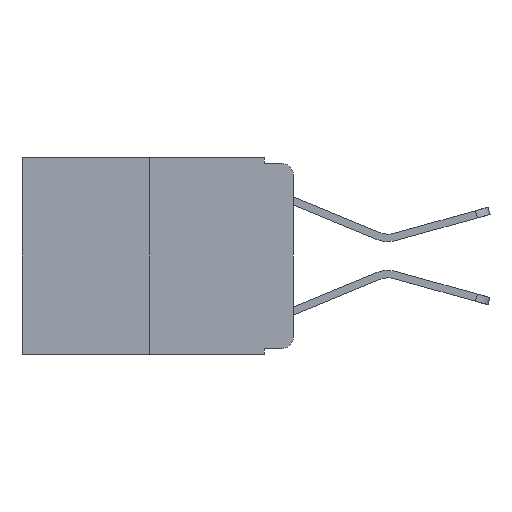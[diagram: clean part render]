
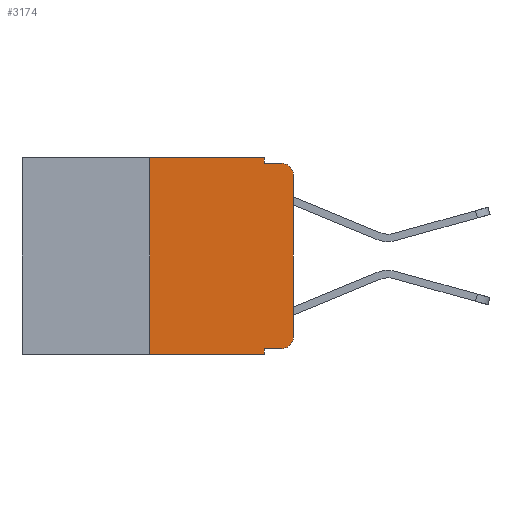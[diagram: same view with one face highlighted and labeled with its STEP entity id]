
A CAD part, left-side view. The second image highlights one B-rep face of the part: STEP entity #3174.
In plain terms, the highlighted planar face has unit normal (-1, 0, 0).
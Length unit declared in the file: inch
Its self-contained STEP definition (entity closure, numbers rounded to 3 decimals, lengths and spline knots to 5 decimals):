
#206 = DIRECTION ( 'NONE',  ( 0., 0., -1. ) ) ;
#505 = ORIENTED_EDGE ( 'NONE', *, *, #9655, .T. ) ;
#578 = VERTEX_POINT ( 'NONE', #1681 ) ;
#584 = CARTESIAN_POINT ( 'NONE',  ( 0., 0.051, -0.343 ) ) ;
#1060 = VERTEX_POINT ( 'NONE', #7971 ) ;
#1079 = LINE ( 'NONE', #1669, #7865 ) ;
#1110 = ORIENTED_EDGE ( 'NONE', *, *, #9670, .T. ) ;
#1277 = VERTEX_POINT ( 'NONE', #584 ) ;
#1289 = VECTOR ( 'NONE', #3260, 39.37008 ) ;
#1319 = DIRECTION ( 'NONE',  ( 0., 0., -1. ) ) ;
#1377 = EDGE_CURVE ( 'NONE', #7410, #1060, #5774, .T. ) ;
#1406 = DIRECTION ( 'NONE',  ( -1., 0., 0. ) ) ;
#1485 = CARTESIAN_POINT ( 'NONE',  ( 0., 0.02, -0.03 ) ) ;
#1519 = VECTOR ( 'NONE', #10667, 39.37008 ) ;
#1527 = CIRCLE ( 'NONE', #7031, 0.02 ) ;
#1564 = LINE ( 'NONE', #7075, #8278 ) ;
#1669 = CARTESIAN_POINT ( 'NONE',  ( 0., 0.051, 0. ) ) ;
#1681 = CARTESIAN_POINT ( 'NONE',  ( 0., 0.051, 0. ) ) ;
#1818 = CARTESIAN_POINT ( 'NONE',  ( 0., 0.02, -0.333 ) ) ;
#2059 = VERTEX_POINT ( 'NONE', #6369 ) ;
#2347 = CARTESIAN_POINT ( 'NONE',  ( 0., 0.02, -0.01 ) ) ;
#2625 = EDGE_CURVE ( 'NONE', #4092, #3668, #1564, .T. ) ;
#2859 = PLANE ( 'NONE',  #4500 ) ;
#3174 = ADVANCED_FACE ( 'NONE', ( #5460 ), #2859, .F. ) ;
#3209 = CARTESIAN_POINT ( 'NONE',  ( 0., 0.051, -0.333 ) ) ;
#3235 = LINE ( 'NONE', #10638, #9751 ) ;
#3260 = DIRECTION ( 'NONE',  ( 0., 0., 1. ) ) ;
#3437 = CIRCLE ( 'NONE', #9424, 0.02 ) ;
#3620 = EDGE_CURVE ( 'NONE', #1060, #3668, #3437, .T. ) ;
#3668 = VERTEX_POINT ( 'NONE', #2347 ) ;
#3849 = EDGE_CURVE ( 'NONE', #578, #4092, #1079, .T. ) ;
#3872 = DIRECTION ( 'NONE',  ( 0., -1., 0. ) ) ;
#4092 = VERTEX_POINT ( 'NONE', #9945 ) ;
#4180 = LINE ( 'NONE', #3209, #8469 ) ;
#4500 = AXIS2_PLACEMENT_3D ( 'NONE', #9171, #6813, #6884 ) ;
#4659 = DIRECTION ( 'NONE',  ( -1., 0., 0. ) ) ;
#4923 = DIRECTION ( 'NONE',  ( 0., -1., 0. ) ) ;
#5192 = ORIENTED_EDGE ( 'NONE', *, *, #3849, .F. ) ;
#5460 = FACE_OUTER_BOUND ( 'NONE', #9489, .T. ) ;
#5604 = ORIENTED_EDGE ( 'NONE', *, *, #9529, .F. ) ;
#5625 = VERTEX_POINT ( 'NONE', #1818 ) ;
#5653 = CARTESIAN_POINT ( 'NONE',  ( 0., 0.25, 0. ) ) ;
#5774 = LINE ( 'NONE', #10717, #1289 ) ;
#5944 = DIRECTION ( 'NONE',  ( 0., 0., -1. ) ) ;
#5953 = DIRECTION ( 'NONE',  ( 0., -1., 0. ) ) ;
#6245 = LINE ( 'NONE', #5653, #1519 ) ;
#6369 = CARTESIAN_POINT ( 'NONE',  ( 0., 0.051, -0.333 ) ) ;
#6577 = CARTESIAN_POINT ( 'NONE',  ( 0., 0., -0.313 ) ) ;
#6813 = DIRECTION ( 'NONE',  ( 1., 0., 0. ) ) ;
#6884 = DIRECTION ( 'NONE',  ( 0., 0., -1. ) ) ;
#6927 = VECTOR ( 'NONE', #3872, 39.37008 ) ;
#7031 = AXIS2_PLACEMENT_3D ( 'NONE', #9723, #4659, #10534 ) ;
#7075 = CARTESIAN_POINT ( 'NONE',  ( 0., 0.051, -0.01 ) ) ;
#7094 = ORIENTED_EDGE ( 'NONE', *, *, #11159, .F. ) ;
#7410 = VERTEX_POINT ( 'NONE', #6577 ) ;
#7642 = ORIENTED_EDGE ( 'NONE', *, *, #8429, .F. ) ;
#7832 = VERTEX_POINT ( 'NONE', #9938 ) ;
#7865 = VECTOR ( 'NONE', #5944, 39.37008 ) ;
#7971 = CARTESIAN_POINT ( 'NONE',  ( 0., 0., -0.03 ) ) ;
#8278 = VECTOR ( 'NONE', #5953, 39.37008 ) ;
#8429 = EDGE_CURVE ( 'NONE', #9460, #7832, #6245, .T. ) ;
#8469 = VECTOR ( 'NONE', #10833, 39.37008 ) ;
#8728 = LINE ( 'NONE', #10791, #8987 ) ;
#8987 = VECTOR ( 'NONE', #4923, 39.37008 ) ;
#9059 = ORIENTED_EDGE ( 'NONE', *, *, #2625, .F. ) ;
#9147 = LINE ( 'NONE', #10565, #6927 ) ;
#9171 = CARTESIAN_POINT ( 'NONE',  ( 0., 0.473, 0. ) ) ;
#9185 = ORIENTED_EDGE ( 'NONE', *, *, #1377, .T. ) ;
#9424 = AXIS2_PLACEMENT_3D ( 'NONE', #1485, #1406, #1319 ) ;
#9460 = VERTEX_POINT ( 'NONE', #9759 ) ;
#9489 = EDGE_LOOP ( 'NONE', ( #9185, #10838, #9059, #5192, #7094, #7642, #505, #5604, #1110, #10089 ) ) ;
#9529 = EDGE_CURVE ( 'NONE', #2059, #1277, #3235, .T. ) ;
#9655 = EDGE_CURVE ( 'NONE', #9460, #1277, #8728, .T. ) ;
#9670 = EDGE_CURVE ( 'NONE', #2059, #5625, #4180, .T. ) ;
#9723 = CARTESIAN_POINT ( 'NONE',  ( 0., 0.02, -0.313 ) ) ;
#9751 = VECTOR ( 'NONE', #206, 39.37008 ) ;
#9759 = CARTESIAN_POINT ( 'NONE',  ( 0., 0.25, -0.343 ) ) ;
#9938 = CARTESIAN_POINT ( 'NONE',  ( 0., 0.25, 0. ) ) ;
#9945 = CARTESIAN_POINT ( 'NONE',  ( 0., 0.051, -0.01 ) ) ;
#10089 = ORIENTED_EDGE ( 'NONE', *, *, #10608, .T. ) ;
#10534 = DIRECTION ( 'NONE',  ( 0., 0., -1. ) ) ;
#10565 = CARTESIAN_POINT ( 'NONE',  ( 0., 0.473, 0. ) ) ;
#10608 = EDGE_CURVE ( 'NONE', #5625, #7410, #1527, .T. ) ;
#10638 = CARTESIAN_POINT ( 'NONE',  ( 0., 0.051, 0. ) ) ;
#10667 = DIRECTION ( 'NONE',  ( 0., 0., 1. ) ) ;
#10717 = CARTESIAN_POINT ( 'NONE',  ( 0., 0., 0. ) ) ;
#10791 = CARTESIAN_POINT ( 'NONE',  ( 0., 0.473, -0.343 ) ) ;
#10833 = DIRECTION ( 'NONE',  ( 0., -1., 0. ) ) ;
#10838 = ORIENTED_EDGE ( 'NONE', *, *, #3620, .T. ) ;
#11159 = EDGE_CURVE ( 'NONE', #7832, #578, #9147, .T. ) ;
